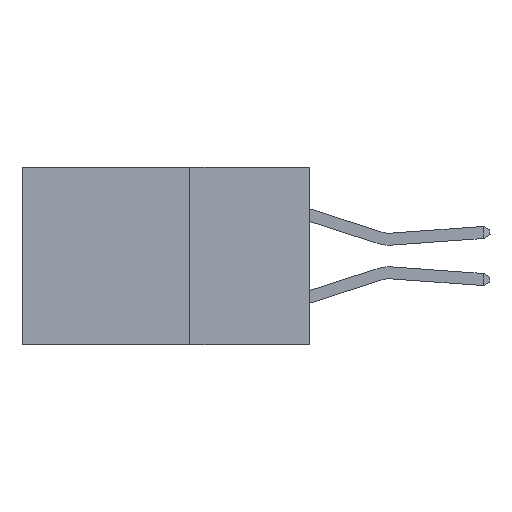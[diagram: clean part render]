
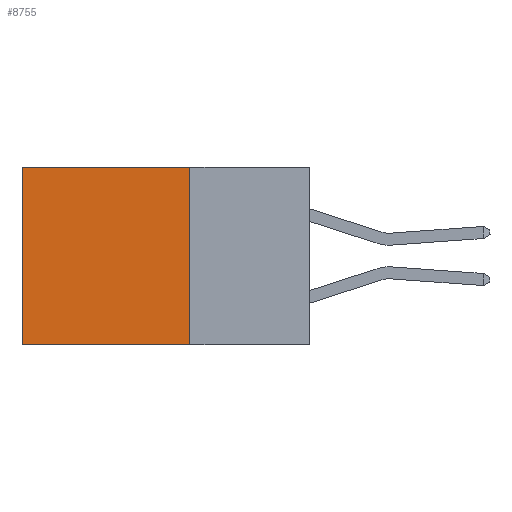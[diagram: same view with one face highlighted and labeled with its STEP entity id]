
A CAD part, left-side view. The second image highlights one B-rep face of the part: STEP entity #8755.
In plain terms, the highlighted planar face has unit normal (-1, 0, 0).
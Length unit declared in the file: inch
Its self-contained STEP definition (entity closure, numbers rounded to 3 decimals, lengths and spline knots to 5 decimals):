
#628 = EDGE_CURVE ( 'NONE', #12066, #12214, #7697, .T. ) ;
#930 = VECTOR ( 'NONE', #3661, 39.37008 ) ;
#1094 = DIRECTION ( 'NONE',  ( 0., 1., 0. ) ) ;
#1888 = EDGE_LOOP ( 'NONE', ( #8447, #6703, #6432, #3276 ) ) ;
#2410 = CARTESIAN_POINT ( 'NONE',  ( 0.2615, 0.25, 0. ) ) ;
#2592 = VECTOR ( 'NONE', #10154, 39.37008 ) ;
#2752 = VECTOR ( 'NONE', #1094, 39.37008 ) ;
#2790 = DIRECTION ( 'NONE',  ( 0., 0., -1. ) ) ;
#2880 = EDGE_CURVE ( 'NONE', #12066, #5606, #5817, .T. ) ;
#3052 = LINE ( 'NONE', #8260, #2592 ) ;
#3170 = DIRECTION ( 'NONE',  ( 1., 0., 0. ) ) ;
#3260 = CARTESIAN_POINT ( 'NONE',  ( 0.2615, 0.6, -0.37 ) ) ;
#3276 = ORIENTED_EDGE ( 'NONE', *, *, #628, .T. ) ;
#3661 = DIRECTION ( 'NONE',  ( 0., 0., -1. ) ) ;
#3795 = VECTOR ( 'NONE', #2790, 39.37008 ) ;
#5165 = VERTEX_POINT ( 'NONE', #3260 ) ;
#5606 = VERTEX_POINT ( 'NONE', #10294 ) ;
#5817 = LINE ( 'NONE', #7851, #930 ) ;
#6312 = CARTESIAN_POINT ( 'NONE',  ( 0.2615, 0.6, 0. ) ) ;
#6339 = CARTESIAN_POINT ( 'NONE',  ( 0.2615, 0.25, -0.37 ) ) ;
#6409 = PLANE ( 'NONE',  #12749 ) ;
#6432 = ORIENTED_EDGE ( 'NONE', *, *, #2880, .F. ) ;
#6444 = EDGE_CURVE ( 'NONE', #12214, #5165, #7114, .T. ) ;
#6703 = ORIENTED_EDGE ( 'NONE', *, *, #11246, .F. ) ;
#7114 = LINE ( 'NONE', #13156, #3795 ) ;
#7697 = LINE ( 'NONE', #9486, #2752 ) ;
#7851 = CARTESIAN_POINT ( 'NONE',  ( 0.2615, 0.25, -0.37 ) ) ;
#8260 = CARTESIAN_POINT ( 'NONE',  ( 0.2615, 0.25, -0.37 ) ) ;
#8447 = ORIENTED_EDGE ( 'NONE', *, *, #6444, .T. ) ;
#8755 = ADVANCED_FACE ( 'NONE', ( #9999 ), #6409, .F. ) ;
#9486 = CARTESIAN_POINT ( 'NONE',  ( 0.2615, 0.25, 0. ) ) ;
#9999 = FACE_OUTER_BOUND ( 'NONE', #1888, .T. ) ;
#10154 = DIRECTION ( 'NONE',  ( 0., 1., 0. ) ) ;
#10294 = CARTESIAN_POINT ( 'NONE',  ( 0.2615, 0.25, -0.37 ) ) ;
#11246 = EDGE_CURVE ( 'NONE', #5606, #5165, #3052, .T. ) ;
#11370 = DIRECTION ( 'NONE',  ( 0., 0., -1. ) ) ;
#12066 = VERTEX_POINT ( 'NONE', #2410 ) ;
#12214 = VERTEX_POINT ( 'NONE', #6312 ) ;
#12749 = AXIS2_PLACEMENT_3D ( 'NONE', #6339, #3170, #11370 ) ;
#13156 = CARTESIAN_POINT ( 'NONE',  ( 0.2615, 0.6, -0.37 ) ) ;
